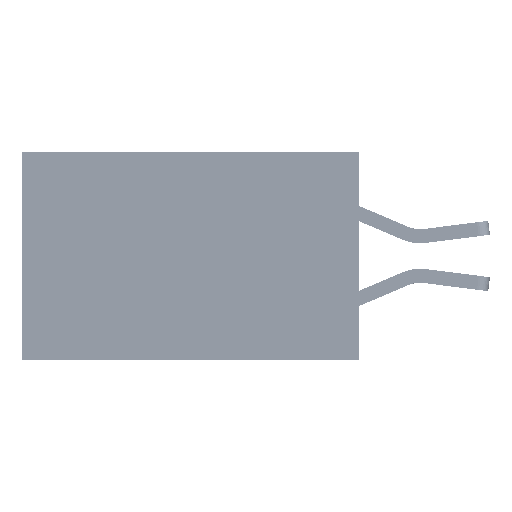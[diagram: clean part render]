
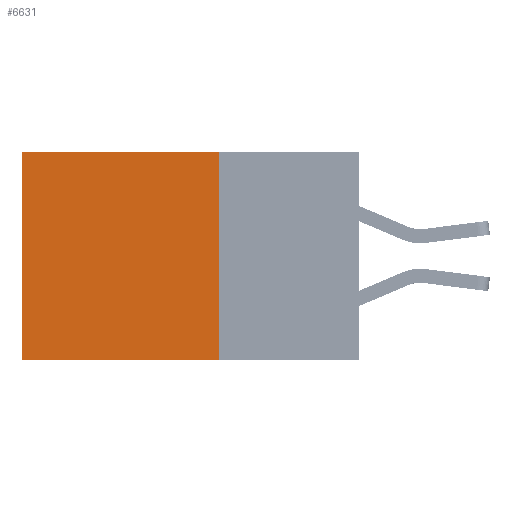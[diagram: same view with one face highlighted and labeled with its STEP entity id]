
A CAD part, left-side view. The second image highlights one B-rep face of the part: STEP entity #6631.
In plain terms, the highlighted planar face has unit normal (-1, 0, 0).
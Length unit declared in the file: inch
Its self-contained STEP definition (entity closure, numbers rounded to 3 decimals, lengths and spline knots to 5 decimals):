
#1516 = EDGE_LOOP ( 'NONE', ( #33322, #42171, #14526, #28410 ) ) ;
#2021 = LINE ( 'NONE', #49181, #44037 ) ;
#2486 = EDGE_CURVE ( 'NONE', #21345, #13877, #23671, .T. ) ;
#2661 = AXIS2_PLACEMENT_3D ( 'NONE', #28473, #4193, #32608 ) ;
#4193 = DIRECTION ( 'NONE',  ( 1., 0., 0. ) ) ;
#5703 = CARTESIAN_POINT ( 'NONE',  ( 0.2875, 0.6, 0. ) ) ;
#6226 = DIRECTION ( 'NONE',  ( 0., 0., -1. ) ) ;
#6631 = ADVANCED_FACE ( 'NONE', ( #17130 ), #24405, .F. ) ;
#7789 = DIRECTION ( 'NONE',  ( 0., 0., -1. ) ) ;
#13877 = VERTEX_POINT ( 'NONE', #42280 ) ;
#14526 = ORIENTED_EDGE ( 'NONE', *, *, #28953, .F. ) ;
#14648 = CARTESIAN_POINT ( 'NONE',  ( 0.2875, 0.25, 0. ) ) ;
#16764 = VECTOR ( 'NONE', #7789, 39.37008 ) ;
#17130 = FACE_OUTER_BOUND ( 'NONE', #1516, .T. ) ;
#19299 = LINE ( 'NONE', #19755, #16764 ) ;
#19755 = CARTESIAN_POINT ( 'NONE',  ( 0.2875, 0.25, 0. ) ) ;
#20210 = CARTESIAN_POINT ( 'NONE',  ( 0.2875, 0.25, -0.37 ) ) ;
#21345 = VERTEX_POINT ( 'NONE', #33940 ) ;
#23671 = LINE ( 'NONE', #5703, #31341 ) ;
#24405 = PLANE ( 'NONE',  #2661 ) ;
#24470 = VERTEX_POINT ( 'NONE', #20210 ) ;
#24790 = DIRECTION ( 'NONE',  ( 0., 1., 0. ) ) ;
#28410 = ORIENTED_EDGE ( 'NONE', *, *, #34908, .T. ) ;
#28473 = CARTESIAN_POINT ( 'NONE',  ( 0.2875, 0.25, 0. ) ) ;
#28953 = EDGE_CURVE ( 'NONE', #33661, #24470, #19299, .T. ) ;
#30086 = EDGE_CURVE ( 'NONE', #24470, #13877, #2021, .T. ) ;
#31341 = VECTOR ( 'NONE', #6226, 39.37008 ) ;
#32608 = DIRECTION ( 'NONE',  ( 0., 0., -1. ) ) ;
#33322 = ORIENTED_EDGE ( 'NONE', *, *, #2486, .T. ) ;
#33661 = VERTEX_POINT ( 'NONE', #14648 ) ;
#33940 = CARTESIAN_POINT ( 'NONE',  ( 0.2875, 0.6, 0. ) ) ;
#34908 = EDGE_CURVE ( 'NONE', #33661, #21345, #39571, .T. ) ;
#39571 = LINE ( 'NONE', #50847, #40870 ) ;
#40870 = VECTOR ( 'NONE', #43017, 39.37008 ) ;
#42171 = ORIENTED_EDGE ( 'NONE', *, *, #30086, .F. ) ;
#42280 = CARTESIAN_POINT ( 'NONE',  ( 0.2875, 0.6, -0.37 ) ) ;
#43017 = DIRECTION ( 'NONE',  ( 0., 1., 0. ) ) ;
#44037 = VECTOR ( 'NONE', #24790, 39.37008 ) ;
#49181 = CARTESIAN_POINT ( 'NONE',  ( 0.2875, 0.25, -0.37 ) ) ;
#50847 = CARTESIAN_POINT ( 'NONE',  ( 0.2875, 0.25, 0. ) ) ;
